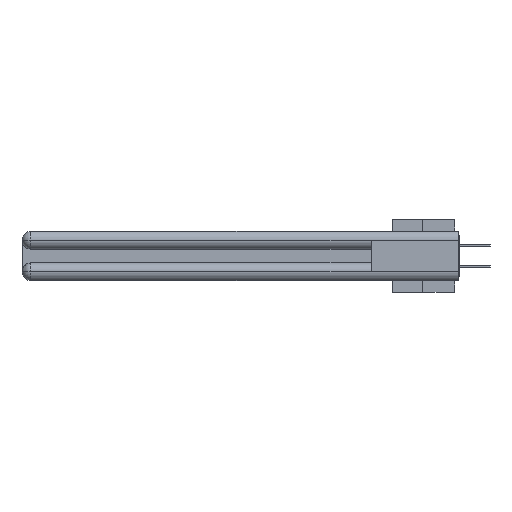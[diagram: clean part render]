
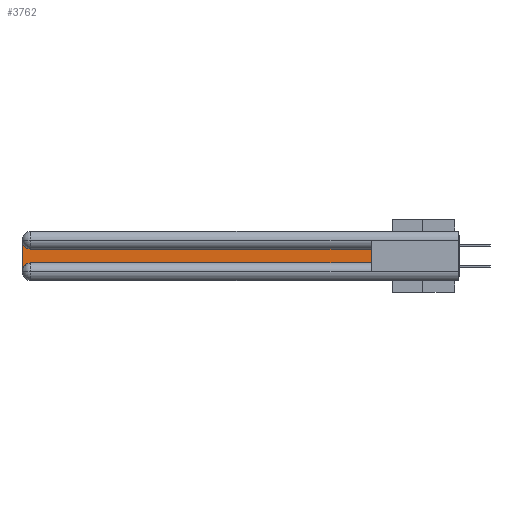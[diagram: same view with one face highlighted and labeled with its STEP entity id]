
A CAD part, left-side view. The second image highlights one B-rep face of the part: STEP entity #3762.
In plain terms, the highlighted planar face has unit normal (-1, 0, 0).
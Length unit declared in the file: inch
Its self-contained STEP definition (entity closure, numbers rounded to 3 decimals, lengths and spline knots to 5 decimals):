
#130 = CARTESIAN_POINT ( 'NONE',  ( 0.075, 3., -0.1225 ) ) ;
#1711 = ORIENTED_EDGE ( 'NONE', *, *, #25295, .T. ) ;
#2922 = CARTESIAN_POINT ( 'NONE',  ( 0.075, 0.6, -0.2175 ) ) ;
#3227 = VECTOR ( 'NONE', #12367, 39.37008 ) ;
#3617 = EDGE_CURVE ( 'NONE', #9769, #9764, #11676, .T. ) ;
#3762 = ADVANCED_FACE ( 'NONE', ( #15779 ), #28896, .F. ) ;
#4208 = LINE ( 'NONE', #11974, #37441 ) ;
#5104 = CARTESIAN_POINT ( 'NONE',  ( 0.075, 0.6, -0.2175 ) ) ;
#5452 = VERTEX_POINT ( 'NONE', #30050 ) ;
#6191 = CARTESIAN_POINT ( 'NONE',  ( 0.075, 2.94, -0.1225 ) ) ;
#6821 = DIRECTION ( 'NONE',  ( 0., 0., -1. ) ) ;
#7228 = DIRECTION ( 'NONE',  ( 1., 0., 0. ) ) ;
#7825 = LINE ( 'NONE', #10086, #29733 ) ;
#9095 = LINE ( 'NONE', #38623, #39984 ) ;
#9764 = VERTEX_POINT ( 'NONE', #5104 ) ;
#9769 = VERTEX_POINT ( 'NONE', #29983 ) ;
#9844 = DIRECTION ( 'NONE',  ( 1., 0., 0. ) ) ;
#10086 = CARTESIAN_POINT ( 'NONE',  ( 0.075, 0.6, -0.1225 ) ) ;
#10523 = CARTESIAN_POINT ( 'NONE',  ( 0.075, 2.94, -0.2775 ) ) ;
#11646 = CARTESIAN_POINT ( 'NONE',  ( 0.075, 3., -0.0625 ) ) ;
#11676 = LINE ( 'NONE', #2922, #3227 ) ;
#11896 = EDGE_LOOP ( 'NONE', ( #28830, #1711, #24284, #40202, #13957, #18514 ) ) ;
#11974 = CARTESIAN_POINT ( 'NONE',  ( 0.075, 3., -0.2175 ) ) ;
#12367 = DIRECTION ( 'NONE',  ( 0., -1., 0. ) ) ;
#12898 = DIRECTION ( 'NONE',  ( 0., 0., -1. ) ) ;
#13957 = ORIENTED_EDGE ( 'NONE', *, *, #3617, .T. ) ;
#14544 = VERTEX_POINT ( 'NONE', #11646 ) ;
#15277 = CARTESIAN_POINT ( 'NONE',  ( 0.075, 3., -0.2775 ) ) ;
#15779 = FACE_OUTER_BOUND ( 'NONE', #11896, .T. ) ;
#15914 = EDGE_CURVE ( 'NONE', #9764, #5452, #9095, .T. ) ;
#16186 = AXIS2_PLACEMENT_3D ( 'NONE', #10523, #16603, #29414 ) ;
#16603 = DIRECTION ( 'NONE',  ( 1., 0., 0. ) ) ;
#17935 = EDGE_CURVE ( 'NONE', #22878, #9769, #26480, .T. ) ;
#18514 = ORIENTED_EDGE ( 'NONE', *, *, #15914, .T. ) ;
#19915 = VERTEX_POINT ( 'NONE', #6191 ) ;
#22878 = VERTEX_POINT ( 'NONE', #15277 ) ;
#22935 = EDGE_CURVE ( 'NONE', #14544, #22878, #4208, .T. ) ;
#24284 = ORIENTED_EDGE ( 'NONE', *, *, #22935, .T. ) ;
#25295 = EDGE_CURVE ( 'NONE', #19915, #14544, #25706, .T. ) ;
#25706 = CIRCLE ( 'NONE', #32092, 0.06 ) ;
#26480 = CIRCLE ( 'NONE', #16186, 0.06 ) ;
#27962 = DIRECTION ( 'NONE',  ( 0., 0., -1. ) ) ;
#28367 = EDGE_CURVE ( 'NONE', #5452, #19915, #7825, .T. ) ;
#28830 = ORIENTED_EDGE ( 'NONE', *, *, #28367, .T. ) ;
#28896 = PLANE ( 'NONE',  #34995 ) ;
#29414 = DIRECTION ( 'NONE',  ( 0., 0., -1. ) ) ;
#29733 = VECTOR ( 'NONE', #38744, 39.37008 ) ;
#29983 = CARTESIAN_POINT ( 'NONE',  ( 0.075, 2.94, -0.2175 ) ) ;
#30050 = CARTESIAN_POINT ( 'NONE',  ( 0.075, 0.6, -0.1225 ) ) ;
#32033 = DIRECTION ( 'NONE',  ( 0., 0., 1. ) ) ;
#32092 = AXIS2_PLACEMENT_3D ( 'NONE', #38575, #7228, #6821 ) ;
#34995 = AXIS2_PLACEMENT_3D ( 'NONE', #130, #9844, #12898 ) ;
#37441 = VECTOR ( 'NONE', #27962, 39.37008 ) ;
#38575 = CARTESIAN_POINT ( 'NONE',  ( 0.075, 2.94, -0.0625 ) ) ;
#38623 = CARTESIAN_POINT ( 'NONE',  ( 0.075, 0.6, -0.2175 ) ) ;
#38744 = DIRECTION ( 'NONE',  ( 0., 1., 0. ) ) ;
#39984 = VECTOR ( 'NONE', #32033, 39.37008 ) ;
#40202 = ORIENTED_EDGE ( 'NONE', *, *, #17935, .T. ) ;
